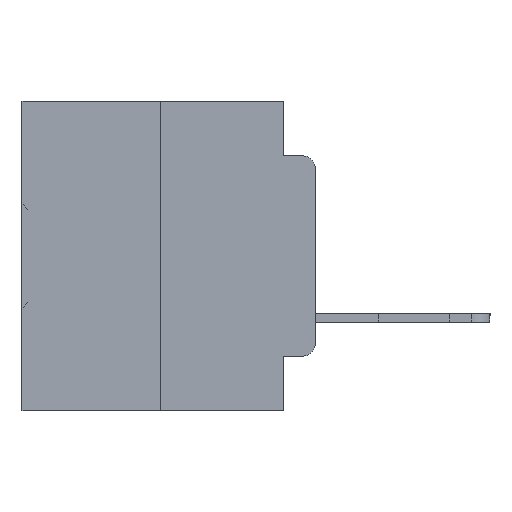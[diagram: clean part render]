
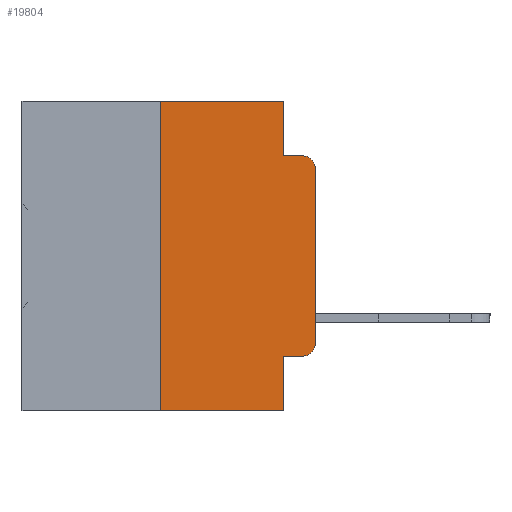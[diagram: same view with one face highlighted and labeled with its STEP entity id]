
A CAD part, left-side view. The second image highlights one B-rep face of the part: STEP entity #19804.
In plain terms, the highlighted planar face has unit normal (-1, 0, 0).
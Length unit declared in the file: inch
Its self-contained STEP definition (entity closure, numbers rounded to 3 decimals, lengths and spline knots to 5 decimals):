
#1024 = CARTESIAN_POINT ( 'NONE',  ( 0., 0.051, -0.4115 ) ) ;
#1417 = ORIENTED_EDGE ( 'NONE', *, *, #3909, .F. ) ;
#1819 = ORIENTED_EDGE ( 'NONE', *, *, #24984, .F. ) ;
#1931 = DIRECTION ( 'NONE',  ( -1., 0., 0. ) ) ;
#1989 = VERTEX_POINT ( 'NONE', #12135 ) ;
#2125 = LINE ( 'NONE', #4337, #7616 ) ;
#2156 = AXIS2_PLACEMENT_3D ( 'NONE', #17940, #1931, #20615 ) ;
#2735 = EDGE_CURVE ( 'NONE', #10292, #24578, #12420, .T. ) ;
#3909 = EDGE_CURVE ( 'NONE', #23462, #1989, #15665, .T. ) ;
#4070 = VECTOR ( 'NONE', #20739, 39.37008 ) ;
#4245 = VECTOR ( 'NONE', #12935, 39.37008 ) ;
#4337 = CARTESIAN_POINT ( 'NONE',  ( 0., 0.051, -0.0885 ) ) ;
#4499 = CARTESIAN_POINT ( 'NONE',  ( 0., 0.051, 0. ) ) ;
#5488 = VERTEX_POINT ( 'NONE', #20795 ) ;
#5561 = EDGE_CURVE ( 'NONE', #30506, #5488, #6867, .T. ) ;
#5937 = LINE ( 'NONE', #1024, #6790 ) ;
#6790 = VECTOR ( 'NONE', #11661, 39.37008 ) ;
#6867 = LINE ( 'NONE', #19646, #27293 ) ;
#7616 = VECTOR ( 'NONE', #17734, 39.37008 ) ;
#7625 = CARTESIAN_POINT ( 'NONE',  ( 0., 0.25, 0. ) ) ;
#7721 = ORIENTED_EDGE ( 'NONE', *, *, #25384, .T. ) ;
#7801 = CARTESIAN_POINT ( 'NONE',  ( 0., 0.051, -0.4115 ) ) ;
#7978 = CARTESIAN_POINT ( 'NONE',  ( 0., 0.051, 0. ) ) ;
#10292 = VERTEX_POINT ( 'NONE', #17451 ) ;
#10575 = ORIENTED_EDGE ( 'NONE', *, *, #2735, .T. ) ;
#10767 = ORIENTED_EDGE ( 'NONE', *, *, #31470, .T. ) ;
#11073 = DIRECTION ( 'NONE',  ( -1., 0., 0. ) ) ;
#11661 = DIRECTION ( 'NONE',  ( 0., -1., 0. ) ) ;
#12135 = CARTESIAN_POINT ( 'NONE',  ( 0., 0.051, -0.0885 ) ) ;
#12153 = DIRECTION ( 'NONE',  ( 0., -1., 0. ) ) ;
#12420 = LINE ( 'NONE', #17317, #24974 ) ;
#12935 = DIRECTION ( 'NONE',  ( 0., 0., 1. ) ) ;
#13340 = DIRECTION ( 'NONE',  ( 1., 0., 0. ) ) ;
#15374 = CIRCLE ( 'NONE', #33329, 0.02 ) ;
#15430 = VERTEX_POINT ( 'NONE', #27129 ) ;
#15665 = LINE ( 'NONE', #32549, #23630 ) ;
#17317 = CARTESIAN_POINT ( 'NONE',  ( 0., 0., 0. ) ) ;
#17324 = CARTESIAN_POINT ( 'NONE',  ( 0., 0.02, -0.0885 ) ) ;
#17451 = CARTESIAN_POINT ( 'NONE',  ( 0., 0., -0.3915 ) ) ;
#17452 = ORIENTED_EDGE ( 'NONE', *, *, #29859, .T. ) ;
#17734 = DIRECTION ( 'NONE',  ( 0., -1., 0. ) ) ;
#17940 = CARTESIAN_POINT ( 'NONE',  ( 0., 0.02, -0.1085 ) ) ;
#18252 = LINE ( 'NONE', #23422, #4070 ) ;
#18274 = ORIENTED_EDGE ( 'NONE', *, *, #5561, .T. ) ;
#18418 = LINE ( 'NONE', #7625, #4245 ) ;
#19646 = CARTESIAN_POINT ( 'NONE',  ( 0., 0.473, -0.5 ) ) ;
#19729 = VECTOR ( 'NONE', #33788, 39.37008 ) ;
#19787 = DIRECTION ( 'NONE',  ( 0., 0., 1. ) ) ;
#19804 = ADVANCED_FACE ( 'NONE', ( #31750 ), #31874, .F. ) ;
#20274 = CARTESIAN_POINT ( 'NONE',  ( 0., 0.25, -0.5 ) ) ;
#20615 = DIRECTION ( 'NONE',  ( 0., 0., -1. ) ) ;
#20739 = DIRECTION ( 'NONE',  ( 0., -1., 0. ) ) ;
#20795 = CARTESIAN_POINT ( 'NONE',  ( 0., 0.051, -0.5 ) ) ;
#20953 = EDGE_CURVE ( 'NONE', #15430, #23462, #18252, .T. ) ;
#21869 = CARTESIAN_POINT ( 'NONE',  ( 0., 0., -0.1085 ) ) ;
#22345 = VERTEX_POINT ( 'NONE', #24360 ) ;
#23422 = CARTESIAN_POINT ( 'NONE',  ( 0., 0.473, 0. ) ) ;
#23462 = VERTEX_POINT ( 'NONE', #7978 ) ;
#23630 = VECTOR ( 'NONE', #32411, 39.37008 ) ;
#24143 = ORIENTED_EDGE ( 'NONE', *, *, #24267, .F. ) ;
#24267 = EDGE_CURVE ( 'NONE', #33997, #5488, #27650, .T. ) ;
#24360 = CARTESIAN_POINT ( 'NONE',  ( 0., 0.02, -0.4115 ) ) ;
#24578 = VERTEX_POINT ( 'NONE', #21869 ) ;
#24829 = EDGE_CURVE ( 'NONE', #1989, #33690, #2125, .T. ) ;
#24974 = VECTOR ( 'NONE', #19787, 39.37008 ) ;
#24984 = EDGE_CURVE ( 'NONE', #30506, #15430, #18418, .T. ) ;
#25384 = EDGE_CURVE ( 'NONE', #24578, #33690, #27984, .T. ) ;
#25713 = EDGE_LOOP ( 'NONE', ( #10575, #7721, #28553, #1417, #29429, #1819, #18274, #24143, #17452, #10767 ) ) ;
#27078 = CARTESIAN_POINT ( 'NONE',  ( 0., 0.02, -0.3915 ) ) ;
#27129 = CARTESIAN_POINT ( 'NONE',  ( 0., 0.25, 0. ) ) ;
#27293 = VECTOR ( 'NONE', #12153, 39.37008 ) ;
#27650 = LINE ( 'NONE', #4499, #19729 ) ;
#27984 = CIRCLE ( 'NONE', #2156, 0.02 ) ;
#28553 = ORIENTED_EDGE ( 'NONE', *, *, #24829, .F. ) ;
#29204 = CARTESIAN_POINT ( 'NONE',  ( 0., 0.473, 0. ) ) ;
#29429 = ORIENTED_EDGE ( 'NONE', *, *, #20953, .F. ) ;
#29748 = DIRECTION ( 'NONE',  ( 0., 0., -1. ) ) ;
#29859 = EDGE_CURVE ( 'NONE', #33997, #22345, #5937, .T. ) ;
#30433 = AXIS2_PLACEMENT_3D ( 'NONE', #29204, #13340, #31996 ) ;
#30506 = VERTEX_POINT ( 'NONE', #20274 ) ;
#31470 = EDGE_CURVE ( 'NONE', #22345, #10292, #15374, .T. ) ;
#31750 = FACE_OUTER_BOUND ( 'NONE', #25713, .T. ) ;
#31874 = PLANE ( 'NONE',  #30433 ) ;
#31996 = DIRECTION ( 'NONE',  ( 0., 0., -1. ) ) ;
#32411 = DIRECTION ( 'NONE',  ( 0., 0., -1. ) ) ;
#32549 = CARTESIAN_POINT ( 'NONE',  ( 0., 0.051, 0. ) ) ;
#33329 = AXIS2_PLACEMENT_3D ( 'NONE', #27078, #11073, #29748 ) ;
#33690 = VERTEX_POINT ( 'NONE', #17324 ) ;
#33788 = DIRECTION ( 'NONE',  ( 0., 0., -1. ) ) ;
#33997 = VERTEX_POINT ( 'NONE', #7801 ) ;
